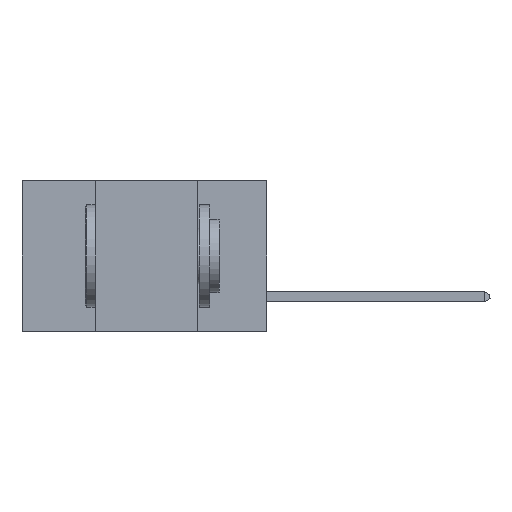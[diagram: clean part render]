
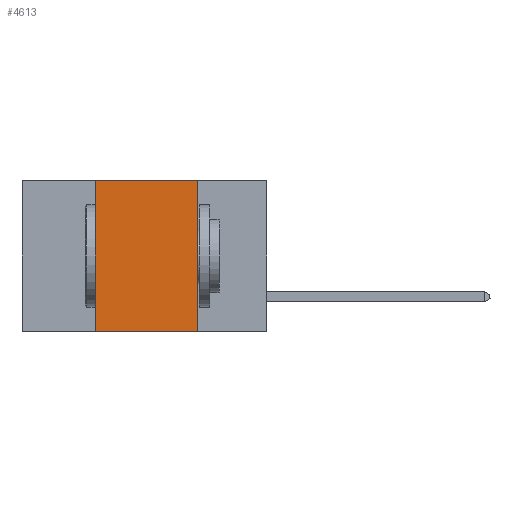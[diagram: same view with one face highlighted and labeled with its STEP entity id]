
A CAD part, left-side view. The second image highlights one B-rep face of the part: STEP entity #4613.
In plain terms, the highlighted planar face has unit normal (-1, 0, 0).
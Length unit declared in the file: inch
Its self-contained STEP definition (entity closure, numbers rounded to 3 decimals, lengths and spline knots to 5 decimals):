
#227 = EDGE_CURVE ( 'NONE', #376, #1623, #1864, .T. ) ;
#376 = VERTEX_POINT ( 'NONE', #3455 ) ;
#685 = EDGE_CURVE ( 'NONE', #376, #2075, #7683, .T. ) ;
#687 = VECTOR ( 'NONE', #4600, 39.37008 ) ;
#1623 = VERTEX_POINT ( 'NONE', #4378 ) ;
#1864 = LINE ( 'NONE', #4868, #5186 ) ;
#2075 = VERTEX_POINT ( 'NONE', #5882 ) ;
#3455 = CARTESIAN_POINT ( 'NONE',  ( 0., 0.42, -0.37 ) ) ;
#3761 = CARTESIAN_POINT ( 'NONE',  ( 0., 0.6, -0.37 ) ) ;
#3792 = EDGE_LOOP ( 'NONE', ( #9120, #8681, #8662, #5675 ) ) ;
#3862 = PLANE ( 'NONE',  #9353 ) ;
#4378 = CARTESIAN_POINT ( 'NONE',  ( 0., 0.42, 0. ) ) ;
#4600 = DIRECTION ( 'NONE',  ( 0., 0., -1. ) ) ;
#4613 = ADVANCED_FACE ( 'NONE', ( #10090 ), #3862, .F. ) ;
#4664 = EDGE_CURVE ( 'NONE', #9178, #2075, #7228, .T. ) ;
#4868 = CARTESIAN_POINT ( 'NONE',  ( 0., 0.42, 0. ) ) ;
#4987 = DIRECTION ( 'NONE',  ( 0., 0., 1. ) ) ;
#5008 = VECTOR ( 'NONE', #8202, 39.37008 ) ;
#5186 = VECTOR ( 'NONE', #4987, 39.37008 ) ;
#5493 = VECTOR ( 'NONE', #6824, 39.37008 ) ;
#5675 = ORIENTED_EDGE ( 'NONE', *, *, #685, .T. ) ;
#5879 = CARTESIAN_POINT ( 'NONE',  ( 0., 0.6, 0. ) ) ;
#5882 = CARTESIAN_POINT ( 'NONE',  ( 0., 0.17, -0.37 ) ) ;
#6483 = DIRECTION ( 'NONE',  ( 1., 0., 0. ) ) ;
#6818 = EDGE_CURVE ( 'NONE', #1623, #9178, #10175, .T. ) ;
#6824 = DIRECTION ( 'NONE',  ( 0., -1., 0. ) ) ;
#7228 = LINE ( 'NONE', #9102, #687 ) ;
#7683 = LINE ( 'NONE', #3761, #5008 ) ;
#8202 = DIRECTION ( 'NONE',  ( 0., -1., 0. ) ) ;
#8662 = ORIENTED_EDGE ( 'NONE', *, *, #227, .F. ) ;
#8681 = ORIENTED_EDGE ( 'NONE', *, *, #6818, .F. ) ;
#9102 = CARTESIAN_POINT ( 'NONE',  ( 0., 0.17, 0. ) ) ;
#9120 = ORIENTED_EDGE ( 'NONE', *, *, #4664, .F. ) ;
#9178 = VERTEX_POINT ( 'NONE', #10450 ) ;
#9353 = AXIS2_PLACEMENT_3D ( 'NONE', #10860, #6483, #9945 ) ;
#9945 = DIRECTION ( 'NONE',  ( 0., 0., -1. ) ) ;
#10090 = FACE_OUTER_BOUND ( 'NONE', #3792, .T. ) ;
#10175 = LINE ( 'NONE', #5879, #5493 ) ;
#10450 = CARTESIAN_POINT ( 'NONE',  ( 0., 0.17, 0. ) ) ;
#10860 = CARTESIAN_POINT ( 'NONE',  ( 0., 0.6, 0. ) ) ;
